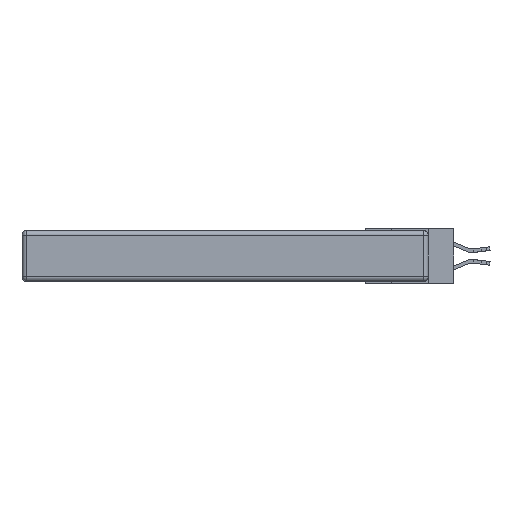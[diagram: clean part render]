
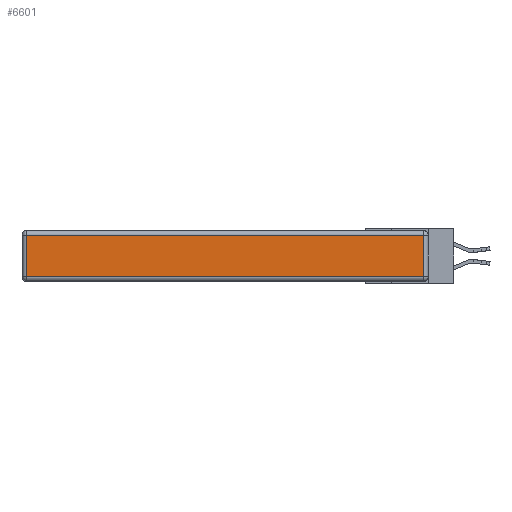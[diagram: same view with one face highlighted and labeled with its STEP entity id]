
A CAD part, left-side view. The second image highlights one B-rep face of the part: STEP entity #6601.
In plain terms, the highlighted planar face has unit normal (-1, 0, 0).
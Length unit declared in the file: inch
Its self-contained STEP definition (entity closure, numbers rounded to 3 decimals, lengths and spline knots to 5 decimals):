
#387 = VECTOR ( 'NONE', #5293, 39.37008 ) ;
#531 = EDGE_LOOP ( 'NONE', ( #8342, #14911, #2550, #2200 ) ) ;
#759 = DIRECTION ( 'NONE',  ( 0., 0., -1. ) ) ;
#1344 = VECTOR ( 'NONE', #3976, 39.37008 ) ;
#1592 = CARTESIAN_POINT ( 'NONE',  ( 0., 0.03, -0.343 ) ) ;
#2200 = ORIENTED_EDGE ( 'NONE', *, *, #12086, .T. ) ;
#2513 = LINE ( 'NONE', #6358, #1344 ) ;
#2550 = ORIENTED_EDGE ( 'NONE', *, *, #12264, .T. ) ;
#3670 = VERTEX_POINT ( 'NONE', #8752 ) ;
#3694 = EDGE_CURVE ( 'NONE', #3670, #9012, #7453, .T. ) ;
#3976 = DIRECTION ( 'NONE',  ( 0., -1., 0. ) ) ;
#4426 = CARTESIAN_POINT ( 'NONE',  ( 0., 2.72, -0.03 ) ) ;
#5293 = DIRECTION ( 'NONE',  ( 0., 0., 1. ) ) ;
#5339 = PLANE ( 'NONE',  #14821 ) ;
#5624 = VERTEX_POINT ( 'NONE', #7630 ) ;
#5904 = VECTOR ( 'NONE', #759, 39.37008 ) ;
#6358 = CARTESIAN_POINT ( 'NONE',  ( 0., 0., -0.313 ) ) ;
#6601 = ADVANCED_FACE ( 'NONE', ( #8265 ), #5339, .T. ) ;
#7240 = EDGE_CURVE ( 'NONE', #5624, #3670, #2513, .T. ) ;
#7453 = LINE ( 'NONE', #1592, #387 ) ;
#7630 = CARTESIAN_POINT ( 'NONE',  ( 0., 2.72, -0.313 ) ) ;
#7777 = DIRECTION ( 'NONE',  ( 0., 0., 1. ) ) ;
#8190 = VERTEX_POINT ( 'NONE', #4426 ) ;
#8265 = FACE_OUTER_BOUND ( 'NONE', #531, .T. ) ;
#8342 = ORIENTED_EDGE ( 'NONE', *, *, #7240, .T. ) ;
#8752 = CARTESIAN_POINT ( 'NONE',  ( 0., 0.03, -0.313 ) ) ;
#8760 = VECTOR ( 'NONE', #10357, 39.37008 ) ;
#9012 = VERTEX_POINT ( 'NONE', #13968 ) ;
#10357 = DIRECTION ( 'NONE',  ( 0., 1., 0. ) ) ;
#12086 = EDGE_CURVE ( 'NONE', #8190, #5624, #14424, .T. ) ;
#12264 = EDGE_CURVE ( 'NONE', #9012, #8190, #15216, .T. ) ;
#13818 = CARTESIAN_POINT ( 'NONE',  ( 0., 0., -0.343 ) ) ;
#13968 = CARTESIAN_POINT ( 'NONE',  ( 0., 0.03, -0.03 ) ) ;
#14400 = CARTESIAN_POINT ( 'NONE',  ( 0., 2.75, -0.03 ) ) ;
#14424 = LINE ( 'NONE', #15406, #5904 ) ;
#14821 = AXIS2_PLACEMENT_3D ( 'NONE', #13818, #15034, #7777 ) ;
#14911 = ORIENTED_EDGE ( 'NONE', *, *, #3694, .T. ) ;
#15034 = DIRECTION ( 'NONE',  ( -1., 0., 0. ) ) ;
#15216 = LINE ( 'NONE', #14400, #8760 ) ;
#15406 = CARTESIAN_POINT ( 'NONE',  ( 0., 2.72, -0.343 ) ) ;
